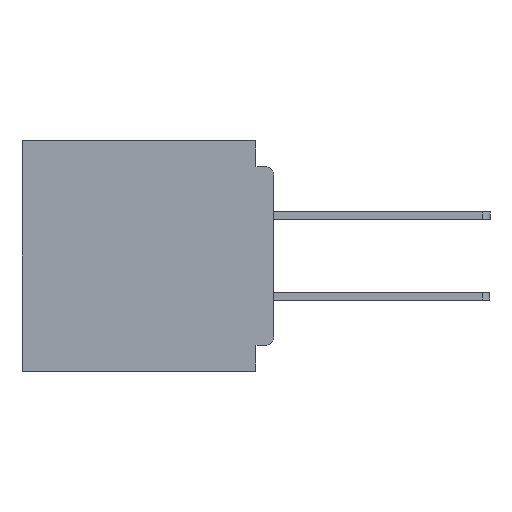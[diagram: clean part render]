
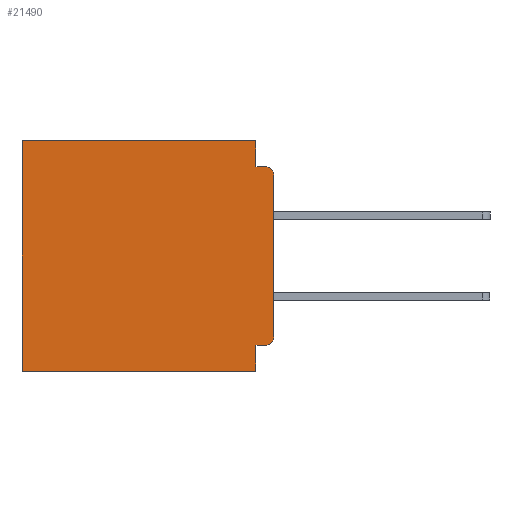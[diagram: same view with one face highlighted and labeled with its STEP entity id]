
A CAD part, left-side view. The second image highlights one B-rep face of the part: STEP entity #21490.
In plain terms, the highlighted planar face has unit normal (-1, 0, 0).
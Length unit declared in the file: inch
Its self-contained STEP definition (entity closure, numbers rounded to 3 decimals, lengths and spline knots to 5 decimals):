
#1090 = CARTESIAN_POINT ( 'NONE',  ( 0.3, 0., -0.045 ) ) ;
#1199 = EDGE_CURVE ( 'NONE', #35622, #2692, #40965, .T. ) ;
#2137 = ORIENTED_EDGE ( 'NONE', *, *, #43096, .F. ) ;
#2608 = CARTESIAN_POINT ( 'NONE',  ( 0.3, 0.015, -0.34 ) ) ;
#2679 = CARTESIAN_POINT ( 'NONE',  ( 0.3, 0., 0. ) ) ;
#2692 = VERTEX_POINT ( 'NONE', #24102 ) ;
#2997 = ORIENTED_EDGE ( 'NONE', *, *, #8687, .F. ) ;
#3174 = PLANE ( 'NONE',  #28640 ) ;
#3227 = LINE ( 'NONE', #18121, #38483 ) ;
#3296 = CARTESIAN_POINT ( 'NONE',  ( 0.3, 0., -0.4 ) ) ;
#3563 = VERTEX_POINT ( 'NONE', #29082 ) ;
#4064 = VECTOR ( 'NONE', #40109, 39.37008 ) ;
#4400 = DIRECTION ( 'NONE',  ( 0., 0., -1. ) ) ;
#4425 = CARTESIAN_POINT ( 'NONE',  ( 0.3, 0.437, 0. ) ) ;
#4774 = VECTOR ( 'NONE', #21930, 39.37008 ) ;
#5148 = ORIENTED_EDGE ( 'NONE', *, *, #19309, .T. ) ;
#5555 = ORIENTED_EDGE ( 'NONE', *, *, #40477, .F. ) ;
#6114 = DIRECTION ( 'NONE',  ( 0., 0., -1. ) ) ;
#6623 = EDGE_LOOP ( 'NONE', ( #2137, #28733, #25545, #39624, #35094, #5148, #5555, #2997, #15781, #36301 ) ) ;
#6991 = LINE ( 'NONE', #1090, #16195 ) ;
#7812 = LINE ( 'NONE', #20484, #24878 ) ;
#8687 = EDGE_CURVE ( 'NONE', #2692, #23652, #13960, .T. ) ;
#9079 = CARTESIAN_POINT ( 'NONE',  ( 0.3, 0.031, 0. ) ) ;
#10156 = DIRECTION ( 'NONE',  ( 0., 0., -1. ) ) ;
#10289 = EDGE_CURVE ( 'NONE', #33100, #34197, #13266, .T. ) ;
#13266 = LINE ( 'NONE', #2679, #4064 ) ;
#13811 = VECTOR ( 'NONE', #32252, 39.37008 ) ;
#13933 = CARTESIAN_POINT ( 'NONE',  ( 0.3, 0.015, -0.06 ) ) ;
#13960 = LINE ( 'NONE', #30888, #21903 ) ;
#14773 = EDGE_CURVE ( 'NONE', #33100, #33879, #7812, .T. ) ;
#14909 = LINE ( 'NONE', #28819, #13811 ) ;
#15781 = ORIENTED_EDGE ( 'NONE', *, *, #1199, .F. ) ;
#16195 = VECTOR ( 'NONE', #18295, 39.37008 ) ;
#16637 = VECTOR ( 'NONE', #17193, 39.37008 ) ;
#17193 = DIRECTION ( 'NONE',  ( 0., 1., 0. ) ) ;
#17378 = DIRECTION ( 'NONE',  ( 0., 0., -1. ) ) ;
#17995 = EDGE_CURVE ( 'NONE', #35622, #36773, #21612, .T. ) ;
#18121 = CARTESIAN_POINT ( 'NONE',  ( 0.3, 0.437, -0.4 ) ) ;
#18295 = DIRECTION ( 'NONE',  ( 0., -1., 0. ) ) ;
#18374 = CARTESIAN_POINT ( 'NONE',  ( 0.3, 0., -0.355 ) ) ;
#18634 = CARTESIAN_POINT ( 'NONE',  ( 0.3, 0.015, -0.045 ) ) ;
#19309 = EDGE_CURVE ( 'NONE', #34197, #36509, #3227, .T. ) ;
#20003 = CARTESIAN_POINT ( 'NONE',  ( 0.3, 0.437, -0.4 ) ) ;
#20484 = CARTESIAN_POINT ( 'NONE',  ( 0.3, 0.031, 0. ) ) ;
#20610 = EDGE_CURVE ( 'NONE', #33879, #43093, #6991, .T. ) ;
#21490 = ADVANCED_FACE ( 'NONE', ( #40928 ), #3174, .F. ) ;
#21612 = CIRCLE ( 'NONE', #36780, 0.015 ) ;
#21903 = VECTOR ( 'NONE', #34177, 39.37008 ) ;
#21930 = DIRECTION ( 'NONE',  ( 0., 1., 0. ) ) ;
#23343 = EDGE_CURVE ( 'NONE', #3563, #43093, #30709, .T. ) ;
#23442 = CARTESIAN_POINT ( 'NONE',  ( 0.3, 0.031, -0.045 ) ) ;
#23652 = VERTEX_POINT ( 'NONE', #35867 ) ;
#23895 = DIRECTION ( 'NONE',  ( 0., 0., -1. ) ) ;
#24102 = CARTESIAN_POINT ( 'NONE',  ( 0.3, 0.031, -0.355 ) ) ;
#24878 = VECTOR ( 'NONE', #23895, 39.37008 ) ;
#25545 = ORIENTED_EDGE ( 'NONE', *, *, #20610, .F. ) ;
#26529 = DIRECTION ( 'NONE',  ( -1., 0., 0. ) ) ;
#28094 = AXIS2_PLACEMENT_3D ( 'NONE', #13933, #37678, #17378 ) ;
#28640 = AXIS2_PLACEMENT_3D ( 'NONE', #43904, #30491, #10156 ) ;
#28733 = ORIENTED_EDGE ( 'NONE', *, *, #23343, .T. ) ;
#28819 = CARTESIAN_POINT ( 'NONE',  ( 0.3, 0., -0.4 ) ) ;
#29082 = CARTESIAN_POINT ( 'NONE',  ( 0.3, 0., -0.06 ) ) ;
#30491 = DIRECTION ( 'NONE',  ( 1., 0., 0. ) ) ;
#30709 = CIRCLE ( 'NONE', #28094, 0.015 ) ;
#30888 = CARTESIAN_POINT ( 'NONE',  ( 0.3, 0.031, -0.4 ) ) ;
#31549 = CARTESIAN_POINT ( 'NONE',  ( 0.3, 0., -0.34 ) ) ;
#32252 = DIRECTION ( 'NONE',  ( 0., 0., -1. ) ) ;
#33100 = VERTEX_POINT ( 'NONE', #9079 ) ;
#33879 = VERTEX_POINT ( 'NONE', #23442 ) ;
#34177 = DIRECTION ( 'NONE',  ( 0., 0., -1. ) ) ;
#34197 = VERTEX_POINT ( 'NONE', #4425 ) ;
#34639 = LINE ( 'NONE', #3296, #16637 ) ;
#35094 = ORIENTED_EDGE ( 'NONE', *, *, #10289, .T. ) ;
#35622 = VERTEX_POINT ( 'NONE', #42125 ) ;
#35867 = CARTESIAN_POINT ( 'NONE',  ( 0.3, 0.031, -0.4 ) ) ;
#36301 = ORIENTED_EDGE ( 'NONE', *, *, #17995, .T. ) ;
#36509 = VERTEX_POINT ( 'NONE', #20003 ) ;
#36773 = VERTEX_POINT ( 'NONE', #31549 ) ;
#36780 = AXIS2_PLACEMENT_3D ( 'NONE', #2608, #26529, #6114 ) ;
#37678 = DIRECTION ( 'NONE',  ( -1., 0., 0. ) ) ;
#38483 = VECTOR ( 'NONE', #4400, 39.37008 ) ;
#39624 = ORIENTED_EDGE ( 'NONE', *, *, #14773, .F. ) ;
#40109 = DIRECTION ( 'NONE',  ( 0., 1., 0. ) ) ;
#40477 = EDGE_CURVE ( 'NONE', #23652, #36509, #34639, .T. ) ;
#40928 = FACE_OUTER_BOUND ( 'NONE', #6623, .T. ) ;
#40965 = LINE ( 'NONE', #18374, #4774 ) ;
#42125 = CARTESIAN_POINT ( 'NONE',  ( 0.3, 0.015, -0.355 ) ) ;
#43093 = VERTEX_POINT ( 'NONE', #18634 ) ;
#43096 = EDGE_CURVE ( 'NONE', #3563, #36773, #14909, .T. ) ;
#43904 = CARTESIAN_POINT ( 'NONE',  ( 0.3, 0., -0.4 ) ) ;
